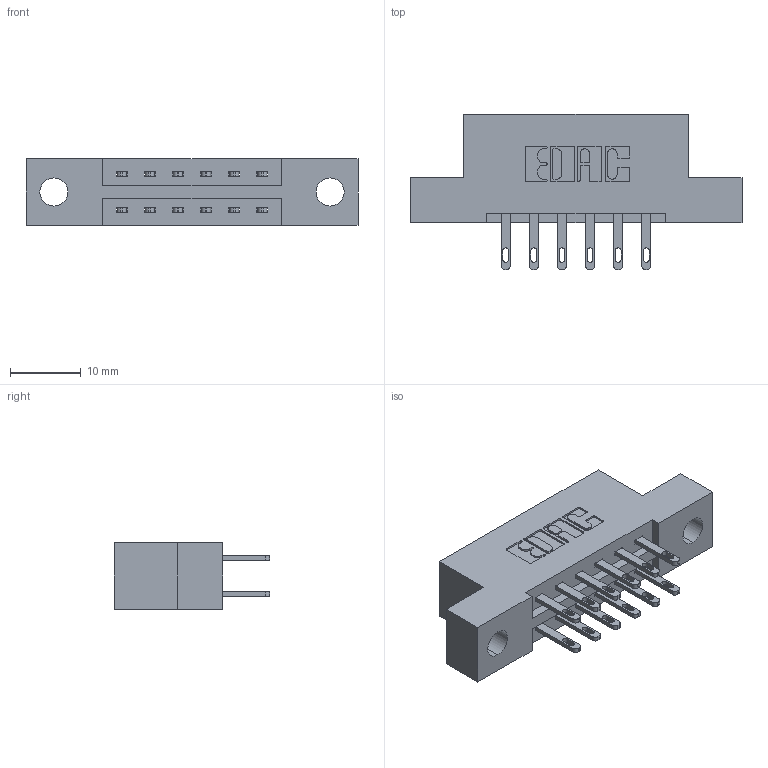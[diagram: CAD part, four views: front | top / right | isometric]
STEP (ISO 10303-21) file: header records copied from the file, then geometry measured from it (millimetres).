
FILE_DESCRIPTION (( 'STEP AP203' ), '1' );
FILE_NAME ('887-012-500-204.STEP', '2020-09-20T16:22:24', ( '' ), ( '' ), 'SwSTEP 2.0', 'SolidWorks 2020', '' );
FILE_SCHEMA (( 'CONFIG_CONTROL_DESIGN' ));
Length unit declared in the file: inch
Products named in the file (3): 887-012-500-204; 345-292-001_345-293-100; 837 Part_Flush Mounting Lugs - 0.156 Dia-TH
Assembly tree (13 placements, depth 2):
  887-012-500-204
    837 Part_Flush Mounting Lugs - 0.156 Dia-TH
    345-292-001_345-293-100  x12
Bounding box: 46.79 x 21.85 x 9.4 mm (x, y, z)
Volume: 4400.4 mm3; surface area: 4555.5 mm2
Topology: 13 solids, 13 shells, 714 faces, 2147 edges, 1430 vertices
Faces by surface type: plane 454, cylinder 260
Entity records: 9241 total; most frequent: CARTESIAN_POINT 1586, ORIENTED_EDGE 1522, DIRECTION 1417, EDGE_CURVE 761, VECTOR 629, LINE 629, VERTEX_POINT 506, AXIS2_PLACEMENT_3D 394
